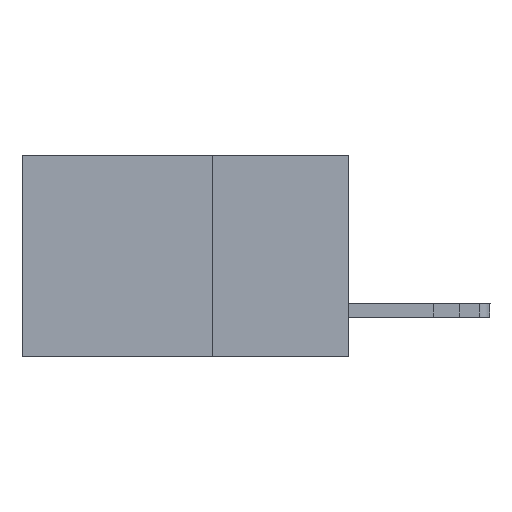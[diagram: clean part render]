
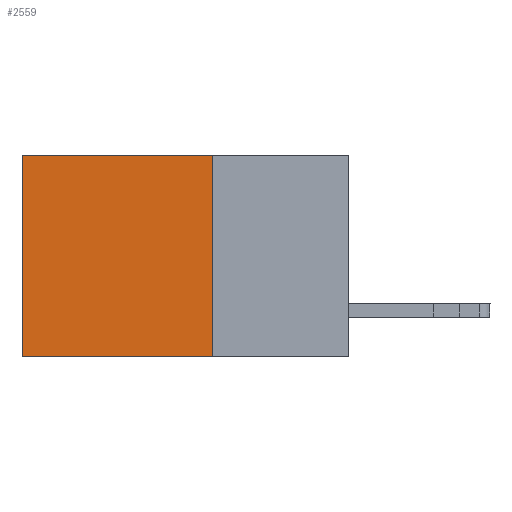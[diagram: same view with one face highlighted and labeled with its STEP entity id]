
A CAD part, left-side view. The second image highlights one B-rep face of the part: STEP entity #2559.
In plain terms, the highlighted planar face has unit normal (-1, 0, 0).
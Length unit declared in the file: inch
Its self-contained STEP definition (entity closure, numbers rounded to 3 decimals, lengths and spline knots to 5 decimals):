
#606 = CARTESIAN_POINT ( 'NONE',  ( 0.2615, 0.25, 0. ) ) ;
#1277 = ORIENTED_EDGE ( 'NONE', *, *, #3114, .T. ) ;
#1308 = ORIENTED_EDGE ( 'NONE', *, *, #6238, .T. ) ;
#1716 = LINE ( 'NONE', #6073, #12171 ) ;
#2463 = DIRECTION ( 'NONE',  ( 1., 0., 0. ) ) ;
#2474 = DIRECTION ( 'NONE',  ( 0., 0., -1. ) ) ;
#2559 = ADVANCED_FACE ( 'NONE', ( #5339 ), #7059, .F. ) ;
#2765 = DIRECTION ( 'NONE',  ( 0., 0., -1. ) ) ;
#2835 = VECTOR ( 'NONE', #3772, 39.37008 ) ;
#2841 = CARTESIAN_POINT ( 'NONE',  ( 0.2615, 0.6, 0. ) ) ;
#3114 = EDGE_CURVE ( 'NONE', #12897, #10654, #1716, .T. ) ;
#3132 = DIRECTION ( 'NONE',  ( 0., 0., -1. ) ) ;
#3772 = DIRECTION ( 'NONE',  ( 0., 1., 0. ) ) ;
#5339 = FACE_OUTER_BOUND ( 'NONE', #11996, .T. ) ;
#5578 = DIRECTION ( 'NONE',  ( 0., 1., 0. ) ) ;
#6073 = CARTESIAN_POINT ( 'NONE',  ( 0.2615, 0.6, -0.37 ) ) ;
#6181 = ORIENTED_EDGE ( 'NONE', *, *, #7767, .F. ) ;
#6238 = EDGE_CURVE ( 'NONE', #6364, #12897, #8260, .T. ) ;
#6364 = VERTEX_POINT ( 'NONE', #7849 ) ;
#7015 = CARTESIAN_POINT ( 'NONE',  ( 0.2615, 0.25, -0.37 ) ) ;
#7059 = PLANE ( 'NONE',  #7568 ) ;
#7552 = EDGE_CURVE ( 'NONE', #9215, #10654, #8227, .T. ) ;
#7568 = AXIS2_PLACEMENT_3D ( 'NONE', #7015, #2463, #2474 ) ;
#7765 = CARTESIAN_POINT ( 'NONE',  ( 0.2615, 0.6, -0.37 ) ) ;
#7767 = EDGE_CURVE ( 'NONE', #6364, #9215, #11066, .T. ) ;
#7849 = CARTESIAN_POINT ( 'NONE',  ( 0.2615, 0.25, 0. ) ) ;
#7932 = VECTOR ( 'NONE', #5578, 39.37008 ) ;
#8197 = CARTESIAN_POINT ( 'NONE',  ( 0.2615, 0.25, -0.37 ) ) ;
#8227 = LINE ( 'NONE', #11932, #2835 ) ;
#8260 = LINE ( 'NONE', #606, #7932 ) ;
#9215 = VERTEX_POINT ( 'NONE', #10315 ) ;
#10315 = CARTESIAN_POINT ( 'NONE',  ( 0.2615, 0.25, -0.37 ) ) ;
#10654 = VERTEX_POINT ( 'NONE', #7765 ) ;
#10753 = VECTOR ( 'NONE', #3132, 39.37008 ) ;
#11066 = LINE ( 'NONE', #8197, #10753 ) ;
#11932 = CARTESIAN_POINT ( 'NONE',  ( 0.2615, 0.25, -0.37 ) ) ;
#11996 = EDGE_LOOP ( 'NONE', ( #1277, #12008, #6181, #1308 ) ) ;
#12008 = ORIENTED_EDGE ( 'NONE', *, *, #7552, .F. ) ;
#12171 = VECTOR ( 'NONE', #2765, 39.37008 ) ;
#12897 = VERTEX_POINT ( 'NONE', #2841 ) ;
